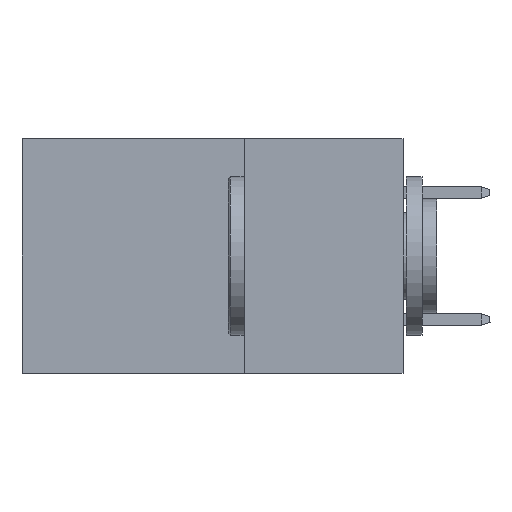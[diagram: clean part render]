
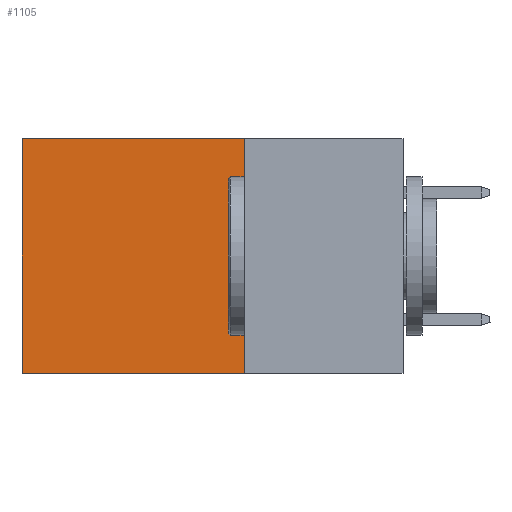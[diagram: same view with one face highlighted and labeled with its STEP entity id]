
A CAD part, left-side view. The second image highlights one B-rep face of the part: STEP entity #1105.
In plain terms, the highlighted planar face has unit normal (-1, 0, 0).
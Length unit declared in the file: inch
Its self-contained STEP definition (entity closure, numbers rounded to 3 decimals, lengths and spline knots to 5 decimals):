
#821 = VECTOR ( 'NONE', #5597, 39.37008 ) ;
#919 = DIRECTION ( 'NONE',  ( 0., 0., -1. ) ) ;
#1105 = ADVANCED_FACE ( 'NONE', ( #17611 ), #17488, .F. ) ;
#1375 = VERTEX_POINT ( 'NONE', #21673 ) ;
#3470 = LINE ( 'NONE', #20224, #22419 ) ;
#3611 = LINE ( 'NONE', #12899, #821 ) ;
#4479 = EDGE_CURVE ( 'NONE', #1375, #11394, #3611, .T. ) ;
#5208 = LINE ( 'NONE', #6845, #15532 ) ;
#5597 = DIRECTION ( 'NONE',  ( 0., 0., -1. ) ) ;
#6138 = EDGE_CURVE ( 'NONE', #9561, #11394, #3470, .T. ) ;
#6152 = VECTOR ( 'NONE', #919, 39.37008 ) ;
#6187 = LINE ( 'NONE', #17602, #6152 ) ;
#6451 = CARTESIAN_POINT ( 'NONE',  ( 0.2875, 0.25, 0. ) ) ;
#6845 = CARTESIAN_POINT ( 'NONE',  ( 0.2875, 0.25, 0. ) ) ;
#7582 = ORIENTED_EDGE ( 'NONE', *, *, #6138, .F. ) ;
#8149 = DIRECTION ( 'NONE',  ( 0., 0., -1. ) ) ;
#9561 = VERTEX_POINT ( 'NONE', #22007 ) ;
#11394 = VERTEX_POINT ( 'NONE', #17826 ) ;
#12899 = CARTESIAN_POINT ( 'NONE',  ( 0.2875, 0.6, 0. ) ) ;
#14026 = DIRECTION ( 'NONE',  ( 1., 0., 0. ) ) ;
#15484 = ORIENTED_EDGE ( 'NONE', *, *, #18157, .T. ) ;
#15532 = VECTOR ( 'NONE', #19845, 39.37008 ) ;
#16042 = ORIENTED_EDGE ( 'NONE', *, *, #22356, .F. ) ;
#17088 = VERTEX_POINT ( 'NONE', #24583 ) ;
#17488 = PLANE ( 'NONE',  #19567 ) ;
#17602 = CARTESIAN_POINT ( 'NONE',  ( 0.2875, 0.25, 0. ) ) ;
#17611 = FACE_OUTER_BOUND ( 'NONE', #19436, .T. ) ;
#17826 = CARTESIAN_POINT ( 'NONE',  ( 0.2875, 0.6, -0.37 ) ) ;
#18157 = EDGE_CURVE ( 'NONE', #17088, #1375, #5208, .T. ) ;
#19436 = EDGE_LOOP ( 'NONE', ( #19706, #7582, #16042, #15484 ) ) ;
#19567 = AXIS2_PLACEMENT_3D ( 'NONE', #6451, #14026, #8149 ) ;
#19706 = ORIENTED_EDGE ( 'NONE', *, *, #4479, .T. ) ;
#19845 = DIRECTION ( 'NONE',  ( 0., 1., 0. ) ) ;
#20224 = CARTESIAN_POINT ( 'NONE',  ( 0.2875, 0.25, -0.37 ) ) ;
#21673 = CARTESIAN_POINT ( 'NONE',  ( 0.2875, 0.6, 0. ) ) ;
#22007 = CARTESIAN_POINT ( 'NONE',  ( 0.2875, 0.25, -0.37 ) ) ;
#22254 = DIRECTION ( 'NONE',  ( 0., 1., 0. ) ) ;
#22356 = EDGE_CURVE ( 'NONE', #17088, #9561, #6187, .T. ) ;
#22419 = VECTOR ( 'NONE', #22254, 39.37008 ) ;
#24583 = CARTESIAN_POINT ( 'NONE',  ( 0.2875, 0.25, 0. ) ) ;
